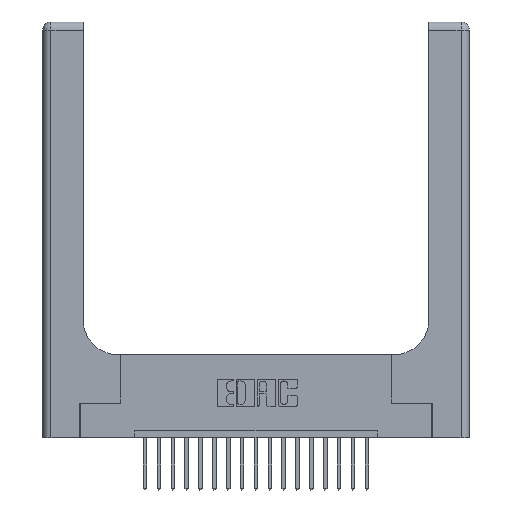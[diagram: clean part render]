
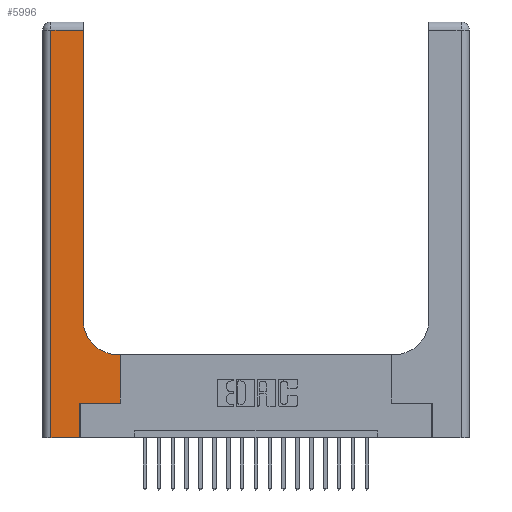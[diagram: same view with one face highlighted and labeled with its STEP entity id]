
A CAD part, top view. The second image highlights one B-rep face of the part: STEP entity #5996.
In plain terms, the highlighted planar face has unit normal (0, 0, 1).
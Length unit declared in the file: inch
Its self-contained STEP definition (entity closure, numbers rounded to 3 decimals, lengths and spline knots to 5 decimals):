
#40 = AXIS2_PLACEMENT_3D ( 'NONE', #2124, #8749, #16914 ) ;
#309 = ORIENTED_EDGE ( 'NONE', *, *, #2926, .T. ) ;
#500 = DIRECTION ( 'NONE',  ( -1., 0., 0. ) ) ;
#576 = DIRECTION ( 'NONE',  ( 0., 1., 0. ) ) ;
#775 = LINE ( 'NONE', #11445, #16992 ) ;
#983 = CARTESIAN_POINT ( 'NONE',  ( 0.06, 0., 0.37 ) ) ;
#1092 = VECTOR ( 'NONE', #9822, 39.37008 ) ;
#2124 = CARTESIAN_POINT ( 'NONE',  ( 0.5415, 0.85, 0.37 ) ) ;
#2910 = VECTOR ( 'NONE', #10256, 39.37008 ) ;
#2926 = EDGE_CURVE ( 'NONE', #9875, #12223, #16567, .T. ) ;
#3594 = CARTESIAN_POINT ( 'NONE',  ( 0.269, 0., 0.37 ) ) ;
#3846 = CARTESIAN_POINT ( 'NONE',  ( 0.5585, 0.25, 0.37 ) ) ;
#3934 = CARTESIAN_POINT ( 'NONE',  ( 0.5585, 0.6, 0.37 ) ) ;
#4242 = VERTEX_POINT ( 'NONE', #5015 ) ;
#4835 = VERTEX_POINT ( 'NONE', #12268 ) ;
#4979 = DIRECTION ( 'NONE',  ( 0., -1., 0. ) ) ;
#5015 = CARTESIAN_POINT ( 'NONE',  ( 0.5585, 0.25, 0.37 ) ) ;
#5150 = EDGE_LOOP ( 'NONE', ( #10876, #12526, #13830, #309, #6337, #21352, #14407, #19417, #15997 ) ) ;
#5996 = ADVANCED_FACE ( 'NONE', ( #8403 ), #11603, .F. ) ;
#6327 = LINE ( 'NONE', #10505, #20219 ) ;
#6337 = ORIENTED_EDGE ( 'NONE', *, *, #8356, .T. ) ;
#6634 = EDGE_CURVE ( 'NONE', #4242, #11900, #12475, .T. ) ;
#6658 = EDGE_CURVE ( 'NONE', #11900, #6956, #6327, .T. ) ;
#6956 = VERTEX_POINT ( 'NONE', #19848 ) ;
#7091 = DIRECTION ( 'NONE',  ( 0., 1., 0. ) ) ;
#7621 = VECTOR ( 'NONE', #576, 39.37008 ) ;
#8104 = CARTESIAN_POINT ( 'NONE',  ( 0., 0., 0.37 ) ) ;
#8356 = EDGE_CURVE ( 'NONE', #12223, #4835, #16244, .T. ) ;
#8403 = FACE_OUTER_BOUND ( 'NONE', #5150, .T. ) ;
#8527 = CARTESIAN_POINT ( 'NONE',  ( 0.2915, 3., 0.37 ) ) ;
#8687 = VERTEX_POINT ( 'NONE', #11674 ) ;
#8749 = DIRECTION ( 'NONE',  ( 0., 0., -1. ) ) ;
#9822 = DIRECTION ( 'NONE',  ( -1., 0., 0. ) ) ;
#9875 = VERTEX_POINT ( 'NONE', #983 ) ;
#10256 = DIRECTION ( 'NONE',  ( 0., 1., 0. ) ) ;
#10505 = CARTESIAN_POINT ( 'NONE',  ( 0.2915, 0.6, 0.37 ) ) ;
#10876 = ORIENTED_EDGE ( 'NONE', *, *, #14376, .T. ) ;
#10941 = DIRECTION ( 'NONE',  ( 1., 0., 0. ) ) ;
#11040 = VECTOR ( 'NONE', #4979, 39.37008 ) ;
#11445 = CARTESIAN_POINT ( 'NONE',  ( 0.269, 0.25, 0.37 ) ) ;
#11529 = DIRECTION ( 'NONE',  ( -1., 0., 0. ) ) ;
#11603 = PLANE ( 'NONE',  #17621 ) ;
#11674 = CARTESIAN_POINT ( 'NONE',  ( 0.2915, 0.85, 0.37 ) ) ;
#11900 = VERTEX_POINT ( 'NONE', #3934 ) ;
#12223 = VERTEX_POINT ( 'NONE', #3594 ) ;
#12268 = CARTESIAN_POINT ( 'NONE',  ( 0.269, 0.25, 0.37 ) ) ;
#12475 = LINE ( 'NONE', #3846, #7621 ) ;
#12526 = ORIENTED_EDGE ( 'NONE', *, *, #13787, .T. ) ;
#13112 = DIRECTION ( 'NONE',  ( 1., 0., 0. ) ) ;
#13553 = EDGE_CURVE ( 'NONE', #6956, #8687, #17054, .T. ) ;
#13787 = EDGE_CURVE ( 'NONE', #19335, #19539, #19379, .T. ) ;
#13830 = ORIENTED_EDGE ( 'NONE', *, *, #15790, .T. ) ;
#14026 = VECTOR ( 'NONE', #10941, 39.37008 ) ;
#14376 = EDGE_CURVE ( 'NONE', #8687, #19335, #15167, .T. ) ;
#14407 = ORIENTED_EDGE ( 'NONE', *, *, #6634, .T. ) ;
#14692 = EDGE_CURVE ( 'NONE', #4835, #4242, #775, .T. ) ;
#15167 = LINE ( 'NONE', #8527, #16741 ) ;
#15275 = CARTESIAN_POINT ( 'NONE',  ( 0.269, 0., 0.37 ) ) ;
#15790 = EDGE_CURVE ( 'NONE', #19539, #9875, #16678, .T. ) ;
#15997 = ORIENTED_EDGE ( 'NONE', *, *, #13553, .T. ) ;
#16244 = LINE ( 'NONE', #15275, #2910 ) ;
#16495 = DIRECTION ( 'NONE',  ( 0., 0., -1. ) ) ;
#16567 = LINE ( 'NONE', #8104, #14026 ) ;
#16678 = LINE ( 'NONE', #21373, #11040 ) ;
#16741 = VECTOR ( 'NONE', #7091, 39.37008 ) ;
#16914 = DIRECTION ( 'NONE',  ( 1., 0., 0. ) ) ;
#16992 = VECTOR ( 'NONE', #13112, 39.37008 ) ;
#17054 = CIRCLE ( 'NONE', #40, 0.25 ) ;
#17621 = AXIS2_PLACEMENT_3D ( 'NONE', #18085, #16495, #11529 ) ;
#17879 = CARTESIAN_POINT ( 'NONE',  ( 0.2915, 2.94, 0.37 ) ) ;
#18085 = CARTESIAN_POINT ( 'NONE',  ( 0., 3., 0.37 ) ) ;
#19335 = VERTEX_POINT ( 'NONE', #17879 ) ;
#19379 = LINE ( 'NONE', #19640, #1092 ) ;
#19417 = ORIENTED_EDGE ( 'NONE', *, *, #6658, .T. ) ;
#19539 = VERTEX_POINT ( 'NONE', #21370 ) ;
#19640 = CARTESIAN_POINT ( 'NONE',  ( 0., 2.94, 0.37 ) ) ;
#19848 = CARTESIAN_POINT ( 'NONE',  ( 0.5415, 0.6, 0.37 ) ) ;
#20219 = VECTOR ( 'NONE', #500, 39.37008 ) ;
#21352 = ORIENTED_EDGE ( 'NONE', *, *, #14692, .T. ) ;
#21370 = CARTESIAN_POINT ( 'NONE',  ( 0.06, 2.94, 0.37 ) ) ;
#21373 = CARTESIAN_POINT ( 'NONE',  ( 0.06, 3., 0.37 ) ) ;
